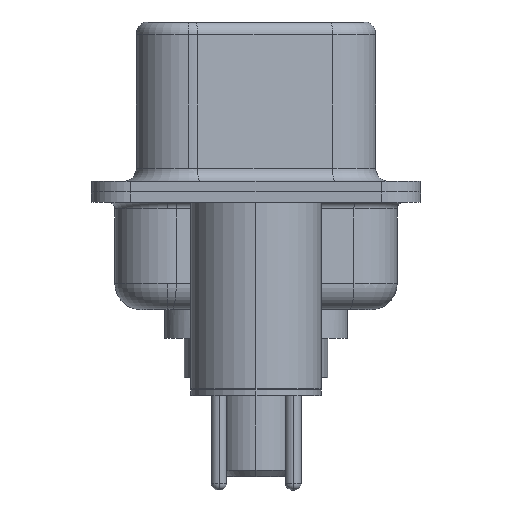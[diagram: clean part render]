
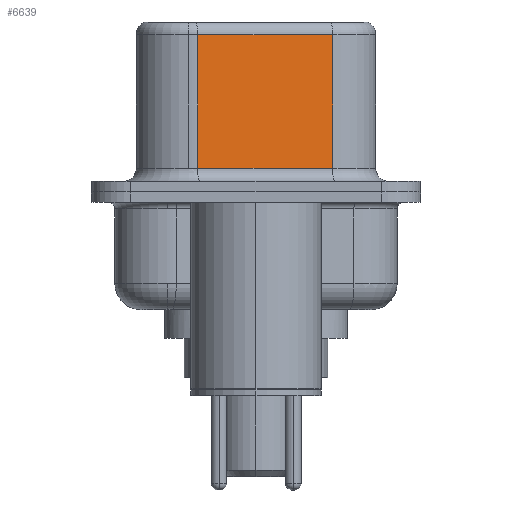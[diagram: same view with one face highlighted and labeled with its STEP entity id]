
A CAD part, left-side view. The second image highlights one B-rep face of the part: STEP entity #6639.
In plain terms, the highlighted planar face has unit normal (-0.985, -0.174, 0).
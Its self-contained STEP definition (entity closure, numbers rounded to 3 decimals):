
#5 = CARTESIAN_POINT ( 'NONE',  ( 4.565, -2.927, 6.52 ) ) ;
#45 = DIRECTION ( 'NONE',  ( 0., 0., -1. ) ) ;
#119 = DIRECTION ( 'NONE',  ( 0., 0., -1. ) ) ;
#1175 = CARTESIAN_POINT ( 'NONE',  ( 4.565, -2.927, 6.52 ) ) ;
#1559 = CARTESIAN_POINT ( 'NONE',  ( 3.655, 2.233, 0.9 ) ) ;
#3662 = DIRECTION ( 'NONE',  ( -0.174, 0.985, 0. ) ) ;
#3788 = VERTEX_POINT ( 'NONE', #12540 ) ;
#3919 = VECTOR ( 'NONE', #13564, 1000. ) ;
#5286 = VERTEX_POINT ( 'NONE', #10034 ) ;
#5720 = VERTEX_POINT ( 'NONE', #9326 ) ;
#6198 = DIRECTION ( 'NONE',  ( -0.174, 0.985, 0. ) ) ;
#6639 = ADVANCED_FACE ( 'NONE', ( #14684 ), #13032, .F. ) ;
#7563 = LINE ( 'NONE', #12172, #3919 ) ;
#7614 = AXIS2_PLACEMENT_3D ( 'NONE', #1175, #15788, #6198 ) ;
#9211 = LINE ( 'NONE', #13972, #16953 ) ;
#9326 = CARTESIAN_POINT ( 'NONE',  ( 4.565, -2.927, 6.02 ) ) ;
#9674 = EDGE_CURVE ( 'NONE', #17624, #5286, #7563, .T. ) ;
#9694 = EDGE_CURVE ( 'NONE', #5720, #5286, #12197, .T. ) ;
#10034 = CARTESIAN_POINT ( 'NONE',  ( 4.565, -2.927, 0.9 ) ) ;
#10629 = CARTESIAN_POINT ( 'NONE',  ( 4.565, -2.927, 6.02 ) ) ;
#10833 = ORIENTED_EDGE ( 'NONE', *, *, #13558, .T. ) ;
#10976 = EDGE_CURVE ( 'NONE', #5720, #3788, #11936, .T. ) ;
#11563 = ORIENTED_EDGE ( 'NONE', *, *, #9694, .F. ) ;
#11936 = LINE ( 'NONE', #10629, #15182 ) ;
#12172 = CARTESIAN_POINT ( 'NONE',  ( 4.565, -2.927, 0.9 ) ) ;
#12197 = LINE ( 'NONE', #5, #14602 ) ;
#12540 = CARTESIAN_POINT ( 'NONE',  ( 3.655, 2.233, 6.02 ) ) ;
#13032 = PLANE ( 'NONE',  #7614 ) ;
#13046 = EDGE_LOOP ( 'NONE', ( #11563, #16300, #10833, #15613 ) ) ;
#13558 = EDGE_CURVE ( 'NONE', #3788, #17624, #9211, .T. ) ;
#13564 = DIRECTION ( 'NONE',  ( 0.174, -0.985, 0. ) ) ;
#13972 = CARTESIAN_POINT ( 'NONE',  ( 3.655, 2.233, 6.52 ) ) ;
#14602 = VECTOR ( 'NONE', #45, 1000. ) ;
#14684 = FACE_OUTER_BOUND ( 'NONE', #13046, .T. ) ;
#15182 = VECTOR ( 'NONE', #3662, 1000. ) ;
#15613 = ORIENTED_EDGE ( 'NONE', *, *, #9674, .T. ) ;
#15788 = DIRECTION ( 'NONE',  ( 0.985, 0.174, 0. ) ) ;
#16300 = ORIENTED_EDGE ( 'NONE', *, *, #10976, .T. ) ;
#16953 = VECTOR ( 'NONE', #119, 1000. ) ;
#17624 = VERTEX_POINT ( 'NONE', #1559 ) ;
